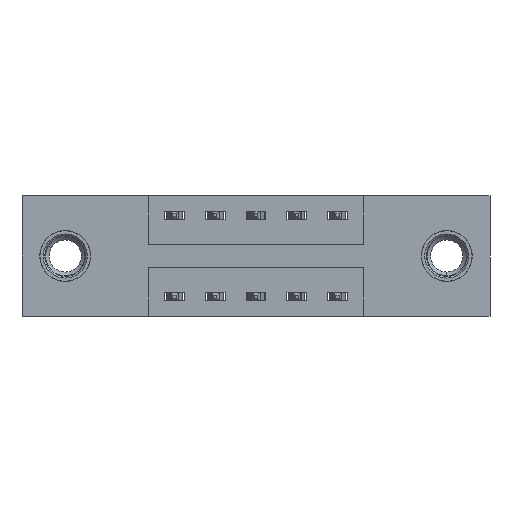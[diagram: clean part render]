
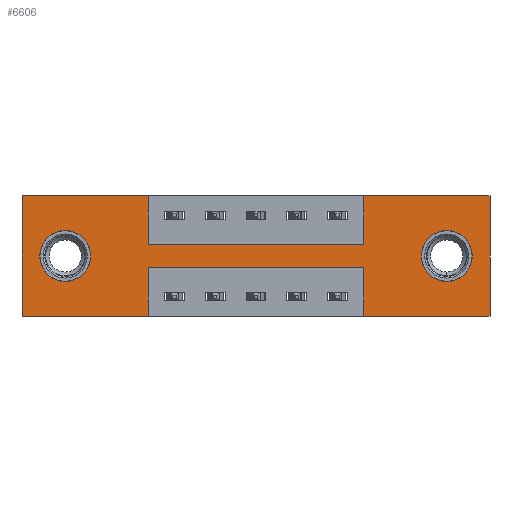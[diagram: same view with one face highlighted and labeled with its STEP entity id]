
A CAD part, front view. The second image highlights one B-rep face of the part: STEP entity #6606.
In plain terms, the highlighted planar face has unit normal (0, -1, 0).
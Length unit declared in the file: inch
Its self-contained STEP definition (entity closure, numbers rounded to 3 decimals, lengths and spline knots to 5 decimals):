
#9 = DIRECTION ( 'NONE',  ( 0., 0., -1. ) ) ;
#17 = CARTESIAN_POINT ( 'NONE',  ( 0.3875, 0., -0.37 ) ) ;
#44 = DIRECTION ( 'NONE',  ( 0., 0., -1. ) ) ;
#56 = LINE ( 'NONE', #2923, #7767 ) ;
#84 = DIRECTION ( 'NONE',  ( 0., 1., 0. ) ) ;
#93 = CARTESIAN_POINT ( 'NONE',  ( 1.3025, 0., -0.185 ) ) ;
#326 = EDGE_LOOP ( 'NONE', ( #7591, #8453 ) ) ;
#360 = AXIS2_PLACEMENT_3D ( 'NONE', #492, #548, #599 ) ;
#395 = CARTESIAN_POINT ( 'NONE',  ( 0.1325, 0., -0.263 ) ) ;
#492 = CARTESIAN_POINT ( 'NONE',  ( 1.3025, 0., -0.185 ) ) ;
#514 = AXIS2_PLACEMENT_3D ( 'NONE', #8633, #8615, #8576 ) ;
#520 = CARTESIAN_POINT ( 'NONE',  ( 0.3875, 0., -0.22 ) ) ;
#548 = DIRECTION ( 'NONE',  ( 0., 1., 0. ) ) ;
#565 = EDGE_CURVE ( 'NONE', #2268, #5648, #8340, .T. ) ;
#599 = DIRECTION ( 'NONE',  ( 0., 0., -1. ) ) ;
#838 = CIRCLE ( 'NONE', #514, 0.078 ) ;
#981 = CARTESIAN_POINT ( 'NONE',  ( 1.0475, 0., 0. ) ) ;
#1052 = AXIS2_PLACEMENT_3D ( 'NONE', #93, #84, #44 ) ;
#1150 = LINE ( 'NONE', #9324, #1270 ) ;
#1270 = VECTOR ( 'NONE', #9293, 39.37008 ) ;
#1378 = VECTOR ( 'NONE', #9017, 39.37008 ) ;
#1433 = LINE ( 'NONE', #5661, #1378 ) ;
#1600 = CARTESIAN_POINT ( 'NONE',  ( 0., 0., -0.37 ) ) ;
#1683 = DIRECTION ( 'NONE',  ( 0., 0., -1. ) ) ;
#1688 = DIRECTION ( 'NONE',  ( 0., -1., 0. ) ) ;
#1715 = PLANE ( 'NONE',  #6303 ) ;
#1754 = DIRECTION ( 'NONE',  ( 0., 0., 1. ) ) ;
#1786 = CARTESIAN_POINT ( 'NONE',  ( 0., 0., -0.37 ) ) ;
#1799 = CARTESIAN_POINT ( 'NONE',  ( 1.0475, 0., -0.37 ) ) ;
#1816 = CARTESIAN_POINT ( 'NONE',  ( 0.1325, 0., -0.107 ) ) ;
#1948 = DIRECTION ( 'NONE',  ( -1., 0., 0. ) ) ;
#1995 = VECTOR ( 'NONE', #5853, 39.37008 ) ;
#2096 = LINE ( 'NONE', #5819, #1995 ) ;
#2198 = VECTOR ( 'NONE', #1948, 39.37008 ) ;
#2268 = VERTEX_POINT ( 'NONE', #8972 ) ;
#2313 = LINE ( 'NONE', #2402, #2198 ) ;
#2402 = CARTESIAN_POINT ( 'NONE',  ( 0.3875, 0., -0.22 ) ) ;
#2490 = CARTESIAN_POINT ( 'NONE',  ( 1.435, 0., 0. ) ) ;
#2496 = VERTEX_POINT ( 'NONE', #8719 ) ;
#2574 = DIRECTION ( 'NONE',  ( 1., 0., 0. ) ) ;
#2647 = VERTEX_POINT ( 'NONE', #981 ) ;
#2712 = VERTEX_POINT ( 'NONE', #5790 ) ;
#2873 = VERTEX_POINT ( 'NONE', #6710 ) ;
#2878 = DIRECTION ( 'NONE',  ( 0., 0., -1. ) ) ;
#2889 = VERTEX_POINT ( 'NONE', #8299 ) ;
#2923 = CARTESIAN_POINT ( 'NONE',  ( 0.3875, 0., -0.15 ) ) ;
#3006 = VERTEX_POINT ( 'NONE', #1816 ) ;
#3291 = EDGE_CURVE ( 'NONE', #9009, #7974, #3991, .T. ) ;
#3500 = DIRECTION ( 'NONE',  ( 0., 0., -1. ) ) ;
#3659 = EDGE_CURVE ( 'NONE', #3006, #9372, #6874, .T. ) ;
#3662 = VECTOR ( 'NONE', #8509, 39.37008 ) ;
#3726 = CARTESIAN_POINT ( 'NONE',  ( 1.435, 0., 0. ) ) ;
#3740 = VECTOR ( 'NONE', #3500, 39.37008 ) ;
#3742 = AXIS2_PLACEMENT_3D ( 'NONE', #6452, #6448, #6434 ) ;
#3902 = LINE ( 'NONE', #17, #7430 ) ;
#3940 = LINE ( 'NONE', #3726, #3740 ) ;
#3991 = LINE ( 'NONE', #1600, #3662 ) ;
#4008 = CIRCLE ( 'NONE', #1052, 0.078 ) ;
#4083 = VECTOR ( 'NONE', #8614, 39.37008 ) ;
#4260 = CARTESIAN_POINT ( 'NONE',  ( 0.3875, 0., 0. ) ) ;
#4274 = EDGE_LOOP ( 'NONE', ( #8300, #8962, #8986, #9013, #9123, #9161, #9347, #8215, #8397, #7795, #4965, #4488 ) ) ;
#4476 = EDGE_CURVE ( 'NONE', #7974, #2496, #4780, .T. ) ;
#4488 = ORIENTED_EDGE ( 'NONE', *, *, #3291, .F. ) ;
#4709 = VECTOR ( 'NONE', #2878, 39.37008 ) ;
#4730 = EDGE_CURVE ( 'NONE', #5717, #2647, #2096, .T. ) ;
#4780 = LINE ( 'NONE', #6582, #4083 ) ;
#4965 = ORIENTED_EDGE ( 'NONE', *, *, #4476, .F. ) ;
#5239 = EDGE_CURVE ( 'NONE', #8642, #2268, #3940, .T. ) ;
#5316 = CARTESIAN_POINT ( 'NONE',  ( 0., 0., -0.37 ) ) ;
#5464 = CARTESIAN_POINT ( 'NONE',  ( 0., 0., -0.37 ) ) ;
#5514 = EDGE_CURVE ( 'NONE', #2496, #2873, #1150, .T. ) ;
#5648 = VERTEX_POINT ( 'NONE', #8290 ) ;
#5661 = CARTESIAN_POINT ( 'NONE',  ( 0., 0., 0. ) ) ;
#5717 = VERTEX_POINT ( 'NONE', #7944 ) ;
#5790 = CARTESIAN_POINT ( 'NONE',  ( 1.3025, 0., -0.107 ) ) ;
#5819 = CARTESIAN_POINT ( 'NONE',  ( 1.0475, 0., 0. ) ) ;
#5853 = DIRECTION ( 'NONE',  ( 0., 0., 1. ) ) ;
#6063 = FACE_BOUND ( 'NONE', #9201, .T. ) ;
#6079 = FACE_BOUND ( 'NONE', #326, .T. ) ;
#6285 = LINE ( 'NONE', #1799, #6529 ) ;
#6303 = AXIS2_PLACEMENT_3D ( 'NONE', #1786, #1688, #1683 ) ;
#6409 = FACE_OUTER_BOUND ( 'NONE', #4274, .T. ) ;
#6434 = DIRECTION ( 'NONE',  ( 0., 0., 1. ) ) ;
#6448 = DIRECTION ( 'NONE',  ( 0., 1., 0. ) ) ;
#6452 = CARTESIAN_POINT ( 'NONE',  ( 0.1325, 0., -0.185 ) ) ;
#6529 = VECTOR ( 'NONE', #1754, 39.37008 ) ;
#6582 = CARTESIAN_POINT ( 'NONE',  ( 0., 0., 0. ) ) ;
#6605 = EDGE_CURVE ( 'NONE', #5648, #2889, #6285, .T. ) ;
#6606 = ADVANCED_FACE ( 'NONE', ( #6063, #6079, #6409 ), #1715, .T. ) ;
#6710 = CARTESIAN_POINT ( 'NONE',  ( 0.3875, 0., 0. ) ) ;
#6779 = EDGE_CURVE ( 'NONE', #2712, #9051, #4008, .T. ) ;
#6874 = CIRCLE ( 'NONE', #3742, 0.078 ) ;
#6959 = EDGE_CURVE ( 'NONE', #2889, #7702, #2313, .T. ) ;
#7013 = EDGE_CURVE ( 'NONE', #2647, #8642, #1433, .T. ) ;
#7142 = CIRCLE ( 'NONE', #360, 0.078 ) ;
#7423 = CARTESIAN_POINT ( 'NONE',  ( 0.3875, 0., -0.15 ) ) ;
#7430 = VECTOR ( 'NONE', #9, 39.37008 ) ;
#7591 = ORIENTED_EDGE ( 'NONE', *, *, #3659, .T. ) ;
#7702 = VERTEX_POINT ( 'NONE', #520 ) ;
#7767 = VECTOR ( 'NONE', #2574, 39.37008 ) ;
#7795 = ORIENTED_EDGE ( 'NONE', *, *, #5514, .F. ) ;
#7944 = CARTESIAN_POINT ( 'NONE',  ( 1.0475, 0., -0.15 ) ) ;
#7974 = VERTEX_POINT ( 'NONE', #5464 ) ;
#7976 = EDGE_CURVE ( 'NONE', #9125, #5717, #56, .T. ) ;
#8204 = VECTOR ( 'NONE', #8997, 39.37008 ) ;
#8215 = ORIENTED_EDGE ( 'NONE', *, *, #7976, .F. ) ;
#8272 = ORIENTED_EDGE ( 'NONE', *, *, #8488, .T. ) ;
#8290 = CARTESIAN_POINT ( 'NONE',  ( 1.0475, 0., -0.37 ) ) ;
#8299 = CARTESIAN_POINT ( 'NONE',  ( 1.0475, 0., -0.22 ) ) ;
#8300 = ORIENTED_EDGE ( 'NONE', *, *, #9351, .F. ) ;
#8340 = LINE ( 'NONE', #5316, #8204 ) ;
#8357 = CARTESIAN_POINT ( 'NONE',  ( 1.3025, 0., -0.263 ) ) ;
#8392 = LINE ( 'NONE', #4260, #4709 ) ;
#8397 = ORIENTED_EDGE ( 'NONE', *, *, #8690, .F. ) ;
#8453 = ORIENTED_EDGE ( 'NONE', *, *, #9035, .T. ) ;
#8488 = EDGE_CURVE ( 'NONE', #9051, #2712, #7142, .T. ) ;
#8509 = DIRECTION ( 'NONE',  ( -1., 0., 0. ) ) ;
#8576 = DIRECTION ( 'NONE',  ( 0., 0., 1. ) ) ;
#8614 = DIRECTION ( 'NONE',  ( 0., 0., 1. ) ) ;
#8615 = DIRECTION ( 'NONE',  ( 0., 1., 0. ) ) ;
#8633 = CARTESIAN_POINT ( 'NONE',  ( 0.1325, 0., -0.185 ) ) ;
#8642 = VERTEX_POINT ( 'NONE', #2490 ) ;
#8690 = EDGE_CURVE ( 'NONE', #2873, #9125, #8392, .T. ) ;
#8719 = CARTESIAN_POINT ( 'NONE',  ( 0., 0., 0. ) ) ;
#8962 = ORIENTED_EDGE ( 'NONE', *, *, #6959, .F. ) ;
#8972 = CARTESIAN_POINT ( 'NONE',  ( 1.435, 0., -0.37 ) ) ;
#8977 = CARTESIAN_POINT ( 'NONE',  ( 0.3875, 0., -0.37 ) ) ;
#8986 = ORIENTED_EDGE ( 'NONE', *, *, #6605, .F. ) ;
#8997 = DIRECTION ( 'NONE',  ( -1., 0., 0. ) ) ;
#9009 = VERTEX_POINT ( 'NONE', #8977 ) ;
#9013 = ORIENTED_EDGE ( 'NONE', *, *, #565, .F. ) ;
#9017 = DIRECTION ( 'NONE',  ( 1., 0., 0. ) ) ;
#9035 = EDGE_CURVE ( 'NONE', #9372, #3006, #838, .T. ) ;
#9051 = VERTEX_POINT ( 'NONE', #8357 ) ;
#9123 = ORIENTED_EDGE ( 'NONE', *, *, #5239, .F. ) ;
#9125 = VERTEX_POINT ( 'NONE', #7423 ) ;
#9161 = ORIENTED_EDGE ( 'NONE', *, *, #7013, .F. ) ;
#9201 = EDGE_LOOP ( 'NONE', ( #9267, #8272 ) ) ;
#9267 = ORIENTED_EDGE ( 'NONE', *, *, #6779, .T. ) ;
#9293 = DIRECTION ( 'NONE',  ( 1., 0., 0. ) ) ;
#9324 = CARTESIAN_POINT ( 'NONE',  ( 0., 0., 0. ) ) ;
#9347 = ORIENTED_EDGE ( 'NONE', *, *, #4730, .F. ) ;
#9351 = EDGE_CURVE ( 'NONE', #7702, #9009, #3902, .T. ) ;
#9372 = VERTEX_POINT ( 'NONE', #395 ) ;
